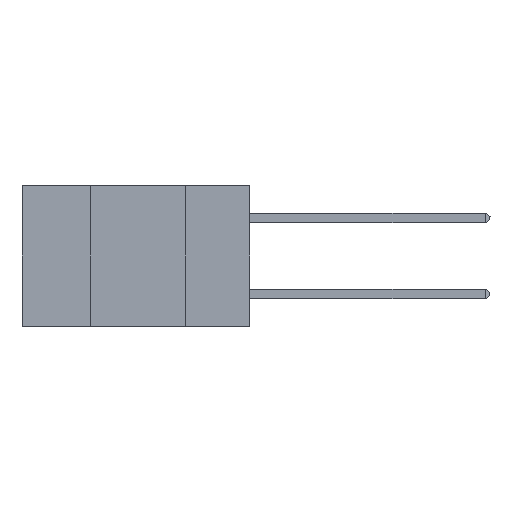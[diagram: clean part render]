
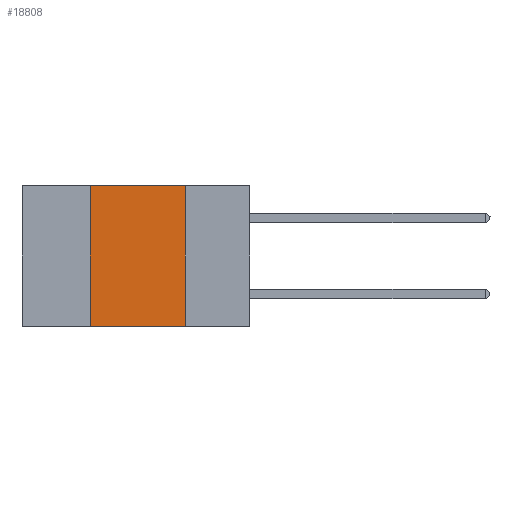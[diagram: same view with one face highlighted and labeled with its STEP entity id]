
A CAD part, left-side view. The second image highlights one B-rep face of the part: STEP entity #18808.
In plain terms, the highlighted planar face has unit normal (-1, 0, 0).
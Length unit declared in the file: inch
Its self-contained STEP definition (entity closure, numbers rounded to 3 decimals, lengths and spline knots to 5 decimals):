
#221 = LINE ( 'NONE', #8427, #19382 ) ;
#899 = PLANE ( 'NONE',  #10706 ) ;
#927 = DIRECTION ( 'NONE',  ( 0., 0., 1. ) ) ;
#945 = LINE ( 'NONE', #9175, #20055 ) ;
#2206 = DIRECTION ( 'NONE',  ( 0., -1., 0. ) ) ;
#2620 = CARTESIAN_POINT ( 'NONE',  ( 0., 0.17, 0. ) ) ;
#2968 = ORIENTED_EDGE ( 'NONE', *, *, #18604, .F. ) ;
#4783 = VERTEX_POINT ( 'NONE', #2620 ) ;
#5794 = VECTOR ( 'NONE', #2206, 39.37008 ) ;
#6071 = CARTESIAN_POINT ( 'NONE',  ( 0., 0.6, -0.37 ) ) ;
#6662 = DIRECTION ( 'NONE',  ( 1., 0., 0. ) ) ;
#6844 = EDGE_CURVE ( 'NONE', #23397, #9606, #19263, .T. ) ;
#6877 = VERTEX_POINT ( 'NONE', #9817 ) ;
#7076 = FACE_OUTER_BOUND ( 'NONE', #21522, .T. ) ;
#8427 = CARTESIAN_POINT ( 'NONE',  ( 0., 0.6, 0. ) ) ;
#9175 = CARTESIAN_POINT ( 'NONE',  ( 0., 0.17, 0. ) ) ;
#9606 = VERTEX_POINT ( 'NONE', #23655 ) ;
#9817 = CARTESIAN_POINT ( 'NONE',  ( 0., 0.42, 0. ) ) ;
#10336 = CARTESIAN_POINT ( 'NONE',  ( 0., 0.42, 0. ) ) ;
#10706 = AXIS2_PLACEMENT_3D ( 'NONE', #13955, #6662, #19455 ) ;
#12821 = DIRECTION ( 'NONE',  ( 0., 0., -1. ) ) ;
#12866 = ORIENTED_EDGE ( 'NONE', *, *, #17106, .F. ) ;
#13008 = DIRECTION ( 'NONE',  ( 0., -1., 0. ) ) ;
#13182 = VECTOR ( 'NONE', #927, 39.37008 ) ;
#13739 = EDGE_CURVE ( 'NONE', #4783, #9606, #945, .T. ) ;
#13955 = CARTESIAN_POINT ( 'NONE',  ( 0., 0.6, 0. ) ) ;
#16564 = ORIENTED_EDGE ( 'NONE', *, *, #13739, .F. ) ;
#17106 = EDGE_CURVE ( 'NONE', #23397, #6877, #22838, .T. ) ;
#17717 = ORIENTED_EDGE ( 'NONE', *, *, #6844, .T. ) ;
#18604 = EDGE_CURVE ( 'NONE', #6877, #4783, #221, .T. ) ;
#18808 = ADVANCED_FACE ( 'NONE', ( #7076 ), #899, .F. ) ;
#19263 = LINE ( 'NONE', #6071, #5794 ) ;
#19382 = VECTOR ( 'NONE', #13008, 39.37008 ) ;
#19455 = DIRECTION ( 'NONE',  ( 0., 0., -1. ) ) ;
#20055 = VECTOR ( 'NONE', #12821, 39.37008 ) ;
#20863 = CARTESIAN_POINT ( 'NONE',  ( 0., 0.42, -0.37 ) ) ;
#21522 = EDGE_LOOP ( 'NONE', ( #16564, #2968, #12866, #17717 ) ) ;
#22838 = LINE ( 'NONE', #10336, #13182 ) ;
#23397 = VERTEX_POINT ( 'NONE', #20863 ) ;
#23655 = CARTESIAN_POINT ( 'NONE',  ( 0., 0.17, -0.37 ) ) ;
